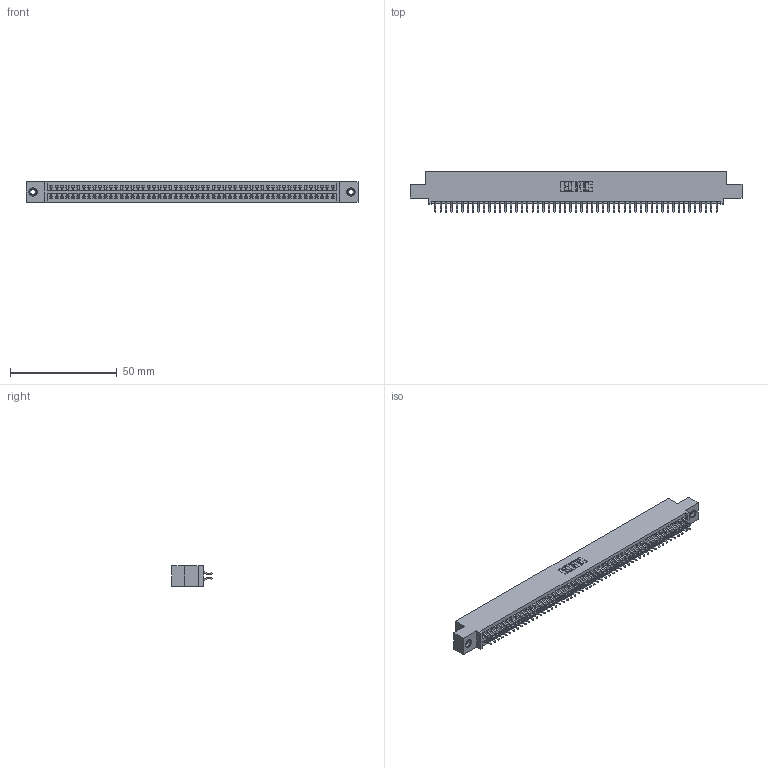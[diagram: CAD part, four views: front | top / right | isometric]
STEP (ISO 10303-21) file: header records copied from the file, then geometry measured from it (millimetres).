
FILE_DESCRIPTION (( 'STEP AP203' ), '1' );
FILE_NAME ('395-106-556-508.STEP', '2019-10-27T06:05:33', ( '' ), ( '' ), 'SwSTEP 2.0', 'SolidWorks 2016', '' );
FILE_SCHEMA (( 'CONFIG_CONTROL_DESIGN' ));
Length unit declared in the file: inch
Products named in the file (4): 345 Part_0.110 Offset - 0.156 Dia-TI; 345-292-001_556 Tail; 345-250-001_345-250-003-102; 395-106-556-508
Assembly tree (109 placements, depth 2):
  395-106-556-508
    345 Part_0.110 Offset - 0.156 Dia-TI
    345-292-001_556 Tail  x106
    345-250-001_345-250-003-102  x2
Bounding box: 155.83 x 19.24 x 9.4 mm (x, y, z)
Volume: 15155.4 mm3; surface area: 22628.8 mm2
Topology: 109 solids, 109 shells, 6126 faces, 18191 edges, 11978 vertices
Faces by surface type: plane 4038, cylinder 2072, cone 12, torus 4
Entity records: 41642 total; most frequent: CARTESIAN_POINT 6967, ORIENTED_EDGE 6882, DIRECTION 6143, EDGE_CURVE 3441, VECTOR 3069, LINE 3069, VERTEX_POINT 2288, AXIS2_PLACEMENT_3D 1537
